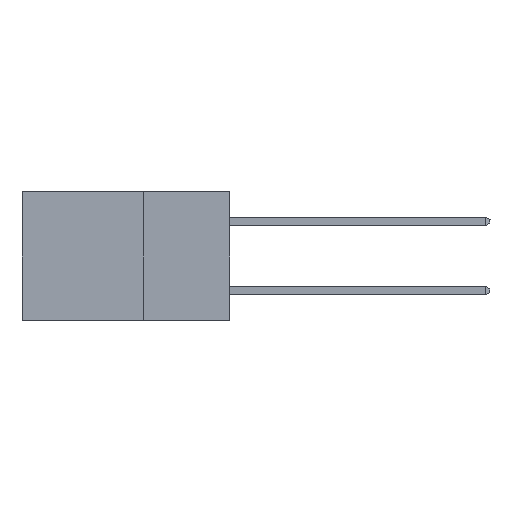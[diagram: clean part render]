
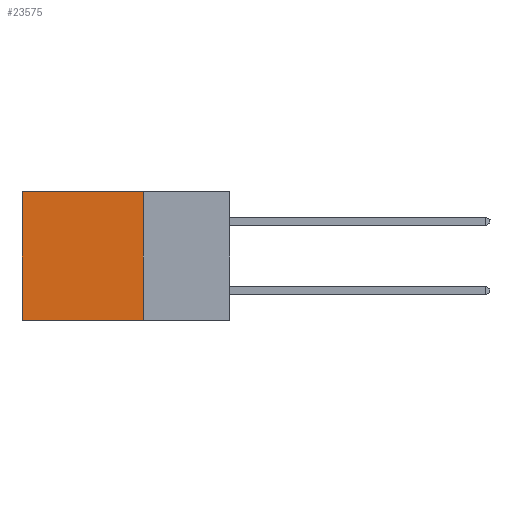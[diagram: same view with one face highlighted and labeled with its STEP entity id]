
A CAD part, left-side view. The second image highlights one B-rep face of the part: STEP entity #23575.
In plain terms, the highlighted planar face has unit normal (-1, 0, 0).
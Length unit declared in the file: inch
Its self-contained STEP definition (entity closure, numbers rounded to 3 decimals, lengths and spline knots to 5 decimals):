
#874 = EDGE_CURVE ( 'NONE', #4511, #1462, #22371, .T. ) ;
#1254 = CARTESIAN_POINT ( 'NONE',  ( 0.2615, 0.25, -0.37 ) ) ;
#1462 = VERTEX_POINT ( 'NONE', #16490 ) ;
#1722 = ORIENTED_EDGE ( 'NONE', *, *, #13967, .T. ) ;
#1814 = AXIS2_PLACEMENT_3D ( 'NONE', #1254, #25659, #3252 ) ;
#2909 = EDGE_CURVE ( 'NONE', #20278, #24632, #22660, .T. ) ;
#3252 = DIRECTION ( 'NONE',  ( 0., 0., -1. ) ) ;
#3923 = VECTOR ( 'NONE', #19786, 39.37008 ) ;
#4511 = VERTEX_POINT ( 'NONE', #25969 ) ;
#7701 = CARTESIAN_POINT ( 'NONE',  ( 0.2615, 0.25, -0.37 ) ) ;
#9587 = PLANE ( 'NONE',  #1814 ) ;
#9891 = DIRECTION ( 'NONE',  ( 0., 1., 0. ) ) ;
#9996 = DIRECTION ( 'NONE',  ( 0., 0., -1. ) ) ;
#11329 = VECTOR ( 'NONE', #13035, 39.37008 ) ;
#13035 = DIRECTION ( 'NONE',  ( 0., 1., 0. ) ) ;
#13967 = EDGE_CURVE ( 'NONE', #24632, #1462, #19573, .T. ) ;
#13980 = CARTESIAN_POINT ( 'NONE',  ( 0.2615, 0.6, -0.37 ) ) ;
#14145 = CARTESIAN_POINT ( 'NONE',  ( 0.2615, 0.25, -0.37 ) ) ;
#14292 = CARTESIAN_POINT ( 'NONE',  ( 0.2615, 0.25, 0. ) ) ;
#14332 = ORIENTED_EDGE ( 'NONE', *, *, #874, .F. ) ;
#14515 = EDGE_LOOP ( 'NONE', ( #1722, #14332, #20884, #20895 ) ) ;
#16490 = CARTESIAN_POINT ( 'NONE',  ( 0.2615, 0.6, -0.37 ) ) ;
#16538 = CARTESIAN_POINT ( 'NONE',  ( 0.2615, 0.25, 0. ) ) ;
#17298 = FACE_OUTER_BOUND ( 'NONE', #14515, .T. ) ;
#17787 = LINE ( 'NONE', #7701, #3923 ) ;
#18669 = CARTESIAN_POINT ( 'NONE',  ( 0.2615, 0.6, 0. ) ) ;
#19573 = LINE ( 'NONE', #13980, #25248 ) ;
#19786 = DIRECTION ( 'NONE',  ( 0., 0., -1. ) ) ;
#20278 = VERTEX_POINT ( 'NONE', #16538 ) ;
#20884 = ORIENTED_EDGE ( 'NONE', *, *, #23873, .F. ) ;
#20895 = ORIENTED_EDGE ( 'NONE', *, *, #2909, .T. ) ;
#22371 = LINE ( 'NONE', #14145, #22513 ) ;
#22513 = VECTOR ( 'NONE', #9891, 39.37008 ) ;
#22660 = LINE ( 'NONE', #14292, #11329 ) ;
#23575 = ADVANCED_FACE ( 'NONE', ( #17298 ), #9587, .F. ) ;
#23873 = EDGE_CURVE ( 'NONE', #20278, #4511, #17787, .T. ) ;
#24632 = VERTEX_POINT ( 'NONE', #18669 ) ;
#25248 = VECTOR ( 'NONE', #9996, 39.37008 ) ;
#25659 = DIRECTION ( 'NONE',  ( 1., 0., 0. ) ) ;
#25969 = CARTESIAN_POINT ( 'NONE',  ( 0.2615, 0.25, -0.37 ) ) ;
